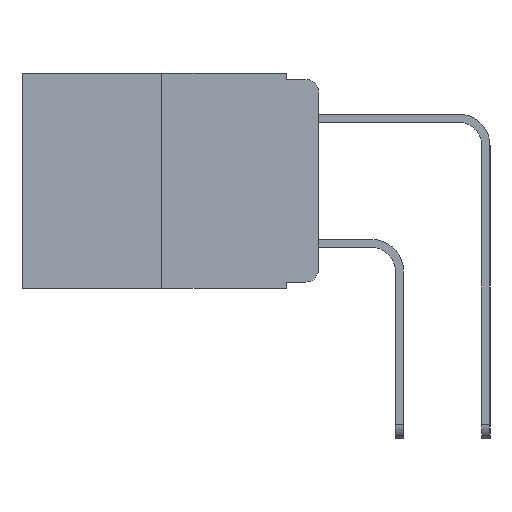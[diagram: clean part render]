
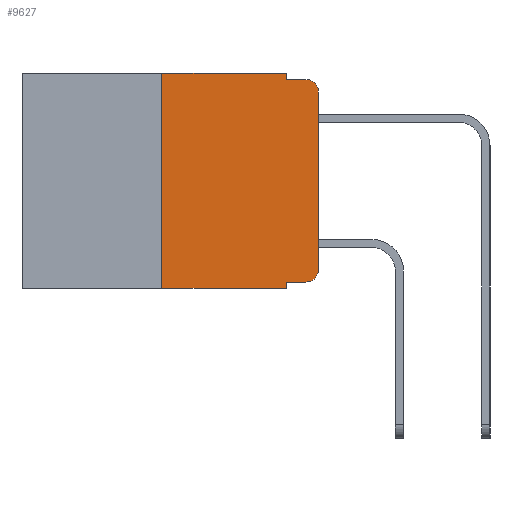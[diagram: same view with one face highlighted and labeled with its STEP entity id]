
A CAD part, left-side view. The second image highlights one B-rep face of the part: STEP entity #9627.
In plain terms, the highlighted planar face has unit normal (-1, 0, 0).
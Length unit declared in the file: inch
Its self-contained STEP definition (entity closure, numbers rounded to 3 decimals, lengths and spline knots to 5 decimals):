
#44 = VERTEX_POINT ( 'NONE', #2085 ) ;
#239 = DIRECTION ( 'NONE',  ( 0., -1., 0. ) ) ;
#508 = DIRECTION ( 'NONE',  ( 0., 0., -1. ) ) ;
#684 = EDGE_CURVE ( 'NONE', #8699, #8862, #10851, .T. ) ;
#868 = CARTESIAN_POINT ( 'NONE',  ( 0., 0., 0. ) ) ;
#1564 = CARTESIAN_POINT ( 'NONE',  ( 0., 0.473, 0. ) ) ;
#1765 = ORIENTED_EDGE ( 'NONE', *, *, #3756, .T. ) ;
#1938 = VECTOR ( 'NONE', #3504, 39.37008 ) ;
#2085 = CARTESIAN_POINT ( 'NONE',  ( 0., 0.051, 0. ) ) ;
#2263 = VERTEX_POINT ( 'NONE', #10694 ) ;
#2288 = AXIS2_PLACEMENT_3D ( 'NONE', #4150, #10568, #12410 ) ;
#2591 = LINE ( 'NONE', #3978, #7632 ) ;
#2714 = EDGE_CURVE ( 'NONE', #2263, #8232, #2591, .T. ) ;
#3020 = LINE ( 'NONE', #10381, #8033 ) ;
#3154 = DIRECTION ( 'NONE',  ( 0., 0., -1. ) ) ;
#3504 = DIRECTION ( 'NONE',  ( 0., -1., 0. ) ) ;
#3573 = DIRECTION ( 'NONE',  ( 0., 0., -1. ) ) ;
#3676 = CARTESIAN_POINT ( 'NONE',  ( 0., 0., -0.313 ) ) ;
#3756 = EDGE_CURVE ( 'NONE', #8668, #8232, #4306, .T. ) ;
#3817 = ORIENTED_EDGE ( 'NONE', *, *, #2714, .F. ) ;
#3908 = CIRCLE ( 'NONE', #9174, 0.02 ) ;
#3978 = CARTESIAN_POINT ( 'NONE',  ( 0., 0.051, -0.01 ) ) ;
#4071 = EDGE_CURVE ( 'NONE', #44, #2263, #10913, .T. ) ;
#4150 = CARTESIAN_POINT ( 'NONE',  ( 0., 0.02, -0.03 ) ) ;
#4306 = CIRCLE ( 'NONE', #2288, 0.02 ) ;
#4491 = DIRECTION ( 'NONE',  ( 0., 0., -1. ) ) ;
#4918 = CARTESIAN_POINT ( 'NONE',  ( 0., 0., -0.03 ) ) ;
#5175 = CARTESIAN_POINT ( 'NONE',  ( 0., 0.02, -0.333 ) ) ;
#5312 = ORIENTED_EDGE ( 'NONE', *, *, #11402, .F. ) ;
#5818 = CARTESIAN_POINT ( 'NONE',  ( 0., 0.473, -0.343 ) ) ;
#5823 = ORIENTED_EDGE ( 'NONE', *, *, #9179, .F. ) ;
#5862 = VECTOR ( 'NONE', #4491, 39.37008 ) ;
#5887 = CARTESIAN_POINT ( 'NONE',  ( 0., 0.473, 0. ) ) ;
#6168 = DIRECTION ( 'NONE',  ( 0., -1., 0. ) ) ;
#6224 = EDGE_CURVE ( 'NONE', #11604, #8862, #7284, .T. ) ;
#6437 = EDGE_CURVE ( 'NONE', #9320, #8668, #12342, .T. ) ;
#6544 = DIRECTION ( 'NONE',  ( -1., 0., 0. ) ) ;
#6576 = VECTOR ( 'NONE', #6168, 39.37008 ) ;
#6743 = VECTOR ( 'NONE', #239, 39.37008 ) ;
#7284 = LINE ( 'NONE', #5818, #1938 ) ;
#7423 = VECTOR ( 'NONE', #7912, 39.37008 ) ;
#7562 = PLANE ( 'NONE',  #10982 ) ;
#7632 = VECTOR ( 'NONE', #9922, 39.37008 ) ;
#7912 = DIRECTION ( 'NONE',  ( 0., 0., 1. ) ) ;
#8007 = CARTESIAN_POINT ( 'NONE',  ( 0., 0.051, 0. ) ) ;
#8033 = VECTOR ( 'NONE', #9480, 39.37008 ) ;
#8232 = VERTEX_POINT ( 'NONE', #11753 ) ;
#8312 = EDGE_CURVE ( 'NONE', #8699, #8449, #9290, .T. ) ;
#8378 = CARTESIAN_POINT ( 'NONE',  ( 0., 0.051, -0.333 ) ) ;
#8449 = VERTEX_POINT ( 'NONE', #5175 ) ;
#8457 = VECTOR ( 'NONE', #3154, 39.37008 ) ;
#8668 = VERTEX_POINT ( 'NONE', #4918 ) ;
#8699 = VERTEX_POINT ( 'NONE', #12168 ) ;
#8862 = VERTEX_POINT ( 'NONE', #12295 ) ;
#8883 = FACE_OUTER_BOUND ( 'NONE', #9324, .T. ) ;
#9174 = AXIS2_PLACEMENT_3D ( 'NONE', #12171, #6544, #508 ) ;
#9179 = EDGE_CURVE ( 'NONE', #11533, #44, #11585, .T. ) ;
#9192 = ORIENTED_EDGE ( 'NONE', *, *, #4071, .F. ) ;
#9290 = LINE ( 'NONE', #8378, #6743 ) ;
#9320 = VERTEX_POINT ( 'NONE', #3676 ) ;
#9324 = EDGE_LOOP ( 'NONE', ( #11616, #1765, #3817, #9192, #5823, #5312, #11787, #12313, #10959, #9769 ) ) ;
#9443 = DIRECTION ( 'NONE',  ( 1., 0., 0. ) ) ;
#9480 = DIRECTION ( 'NONE',  ( 0., 0., 1. ) ) ;
#9608 = EDGE_CURVE ( 'NONE', #8449, #9320, #3908, .T. ) ;
#9627 = ADVANCED_FACE ( 'NONE', ( #8883 ), #7562, .F. ) ;
#9769 = ORIENTED_EDGE ( 'NONE', *, *, #9608, .T. ) ;
#9922 = DIRECTION ( 'NONE',  ( 0., -1., 0. ) ) ;
#10381 = CARTESIAN_POINT ( 'NONE',  ( 0., 0.25, 0. ) ) ;
#10568 = DIRECTION ( 'NONE',  ( -1., 0., 0. ) ) ;
#10694 = CARTESIAN_POINT ( 'NONE',  ( 0., 0.051, -0.01 ) ) ;
#10701 = CARTESIAN_POINT ( 'NONE',  ( 0., 0.25, -0.343 ) ) ;
#10851 = LINE ( 'NONE', #11680, #8457 ) ;
#10913 = LINE ( 'NONE', #8007, #5862 ) ;
#10959 = ORIENTED_EDGE ( 'NONE', *, *, #8312, .T. ) ;
#10982 = AXIS2_PLACEMENT_3D ( 'NONE', #1564, #9443, #3573 ) ;
#11402 = EDGE_CURVE ( 'NONE', #11604, #11533, #3020, .T. ) ;
#11533 = VERTEX_POINT ( 'NONE', #11562 ) ;
#11562 = CARTESIAN_POINT ( 'NONE',  ( 0., 0.25, 0. ) ) ;
#11585 = LINE ( 'NONE', #5887, #6576 ) ;
#11604 = VERTEX_POINT ( 'NONE', #10701 ) ;
#11616 = ORIENTED_EDGE ( 'NONE', *, *, #6437, .T. ) ;
#11680 = CARTESIAN_POINT ( 'NONE',  ( 0., 0.051, 0. ) ) ;
#11753 = CARTESIAN_POINT ( 'NONE',  ( 0., 0.02, -0.01 ) ) ;
#11787 = ORIENTED_EDGE ( 'NONE', *, *, #6224, .T. ) ;
#12168 = CARTESIAN_POINT ( 'NONE',  ( 0., 0.051, -0.333 ) ) ;
#12171 = CARTESIAN_POINT ( 'NONE',  ( 0., 0.02, -0.313 ) ) ;
#12295 = CARTESIAN_POINT ( 'NONE',  ( 0., 0.051, -0.343 ) ) ;
#12313 = ORIENTED_EDGE ( 'NONE', *, *, #684, .F. ) ;
#12342 = LINE ( 'NONE', #868, #7423 ) ;
#12410 = DIRECTION ( 'NONE',  ( 0., 0., -1. ) ) ;
